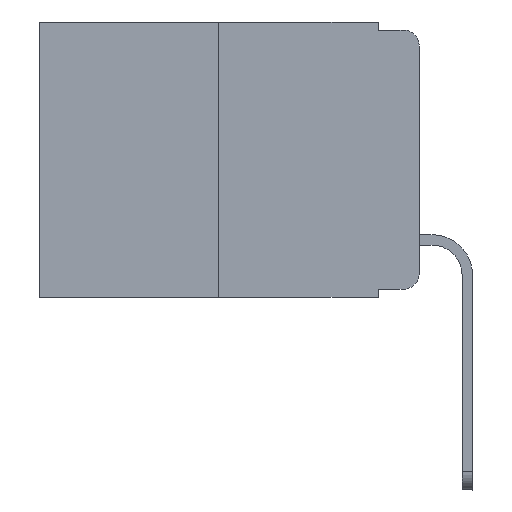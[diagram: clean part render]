
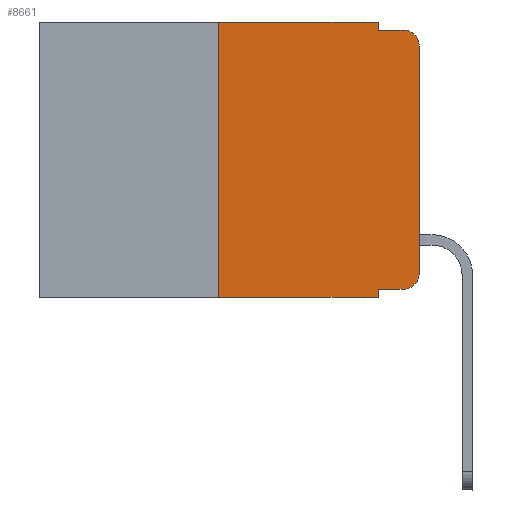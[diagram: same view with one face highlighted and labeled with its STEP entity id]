
A CAD part, left-side view. The second image highlights one B-rep face of the part: STEP entity #8661.
In plain terms, the highlighted planar face has unit normal (-1, 0, 0).
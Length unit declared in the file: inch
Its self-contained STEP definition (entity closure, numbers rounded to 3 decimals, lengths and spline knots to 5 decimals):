
#379 = EDGE_CURVE ( 'NONE', #13050, #4646, #15359, .T. ) ;
#973 = CARTESIAN_POINT ( 'NONE',  ( 0., 0., 0. ) ) ;
#1935 = ORIENTED_EDGE ( 'NONE', *, *, #5807, .F. ) ;
#2223 = ORIENTED_EDGE ( 'NONE', *, *, #12025, .T. ) ;
#2248 = CARTESIAN_POINT ( 'NONE',  ( 0., 0.051, -0.343 ) ) ;
#2332 = EDGE_CURVE ( 'NONE', #15812, #16675, #16079, .T. ) ;
#2363 = VERTEX_POINT ( 'NONE', #13544 ) ;
#3684 = EDGE_CURVE ( 'NONE', #21556, #7158, #5699, .T. ) ;
#3735 = CARTESIAN_POINT ( 'NONE',  ( 0., 0.473, 0. ) ) ;
#3888 = CARTESIAN_POINT ( 'NONE',  ( 0., 0.25, 0. ) ) ;
#4282 = VECTOR ( 'NONE', #18443, 39.37008 ) ;
#4646 = VERTEX_POINT ( 'NONE', #17001 ) ;
#5128 = CARTESIAN_POINT ( 'NONE',  ( 0., 0.25, -0.343 ) ) ;
#5597 = ORIENTED_EDGE ( 'NONE', *, *, #13949, .T. ) ;
#5699 = LINE ( 'NONE', #16818, #9567 ) ;
#5807 = EDGE_CURVE ( 'NONE', #2363, #13050, #10946, .T. ) ;
#5901 = CARTESIAN_POINT ( 'NONE',  ( 0., 0., -0.313 ) ) ;
#6930 = CIRCLE ( 'NONE', #9667, 0.02 ) ;
#7158 = VERTEX_POINT ( 'NONE', #9738 ) ;
#7371 = LINE ( 'NONE', #9457, #11361 ) ;
#7432 = DIRECTION ( 'NONE',  ( 0., 0., -1. ) ) ;
#7552 = DIRECTION ( 'NONE',  ( 0., 0., -1. ) ) ;
#8470 = VERTEX_POINT ( 'NONE', #10294 ) ;
#8509 = LINE ( 'NONE', #16039, #22608 ) ;
#8661 = ADVANCED_FACE ( 'NONE', ( #16834 ), #22338, .F. ) ;
#8668 = CARTESIAN_POINT ( 'NONE',  ( 0., 0.473, -0.343 ) ) ;
#9206 = ORIENTED_EDGE ( 'NONE', *, *, #379, .F. ) ;
#9457 = CARTESIAN_POINT ( 'NONE',  ( 0., 0.473, 0. ) ) ;
#9478 = VERTEX_POINT ( 'NONE', #3888 ) ;
#9567 = VECTOR ( 'NONE', #11366, 39.37008 ) ;
#9667 = AXIS2_PLACEMENT_3D ( 'NONE', #17781, #19611, #21569 ) ;
#9738 = CARTESIAN_POINT ( 'NONE',  ( 0., 0.02, -0.333 ) ) ;
#10294 = CARTESIAN_POINT ( 'NONE',  ( 0., 0., -0.03 ) ) ;
#10668 = VECTOR ( 'NONE', #16191, 39.37008 ) ;
#10749 = ORIENTED_EDGE ( 'NONE', *, *, #21478, .F. ) ;
#10913 = LINE ( 'NONE', #15093, #4282 ) ;
#10946 = LINE ( 'NONE', #16886, #16361 ) ;
#11163 = VECTOR ( 'NONE', #11833, 39.37008 ) ;
#11361 = VECTOR ( 'NONE', #14888, 39.37008 ) ;
#11366 = DIRECTION ( 'NONE',  ( 0., -1., 0. ) ) ;
#11609 = CARTESIAN_POINT ( 'NONE',  ( 0., 0.02, -0.313 ) ) ;
#11772 = DIRECTION ( 'NONE',  ( 0., -1., 0. ) ) ;
#11833 = DIRECTION ( 'NONE',  ( 0., 0., 1. ) ) ;
#12025 = EDGE_CURVE ( 'NONE', #7158, #15551, #13593, .T. ) ;
#12146 = CARTESIAN_POINT ( 'NONE',  ( 0., 0.051, -0.01 ) ) ;
#12442 = DIRECTION ( 'NONE',  ( 0., 0., 1. ) ) ;
#12834 = EDGE_CURVE ( 'NONE', #15812, #9478, #8509, .T. ) ;
#13050 = VERTEX_POINT ( 'NONE', #12146 ) ;
#13519 = VECTOR ( 'NONE', #11772, 39.37008 ) ;
#13544 = CARTESIAN_POINT ( 'NONE',  ( 0., 0.051, 0. ) ) ;
#13593 = CIRCLE ( 'NONE', #16760, 0.02 ) ;
#13949 = EDGE_CURVE ( 'NONE', #8470, #4646, #6930, .T. ) ;
#14345 = ORIENTED_EDGE ( 'NONE', *, *, #2332, .T. ) ;
#14888 = DIRECTION ( 'NONE',  ( 0., -1., 0. ) ) ;
#14961 = DIRECTION ( 'NONE',  ( 1., 0., 0. ) ) ;
#15014 = DIRECTION ( 'NONE',  ( 0., 0., -1. ) ) ;
#15093 = CARTESIAN_POINT ( 'NONE',  ( 0., 0.051, 0. ) ) ;
#15261 = EDGE_CURVE ( 'NONE', #15551, #8470, #15805, .T. ) ;
#15359 = LINE ( 'NONE', #22860, #13519 ) ;
#15551 = VERTEX_POINT ( 'NONE', #5901 ) ;
#15805 = LINE ( 'NONE', #973, #11163 ) ;
#15812 = VERTEX_POINT ( 'NONE', #5128 ) ;
#16039 = CARTESIAN_POINT ( 'NONE',  ( 0., 0.25, 0. ) ) ;
#16079 = LINE ( 'NONE', #8668, #10668 ) ;
#16191 = DIRECTION ( 'NONE',  ( 0., -1., 0. ) ) ;
#16223 = ORIENTED_EDGE ( 'NONE', *, *, #12834, .F. ) ;
#16361 = VECTOR ( 'NONE', #15014, 39.37008 ) ;
#16675 = VERTEX_POINT ( 'NONE', #2248 ) ;
#16760 = AXIS2_PLACEMENT_3D ( 'NONE', #11609, #17197, #7432 ) ;
#16818 = CARTESIAN_POINT ( 'NONE',  ( 0., 0.051, -0.333 ) ) ;
#16834 = FACE_OUTER_BOUND ( 'NONE', #23522, .T. ) ;
#16886 = CARTESIAN_POINT ( 'NONE',  ( 0., 0.051, 0. ) ) ;
#17001 = CARTESIAN_POINT ( 'NONE',  ( 0., 0.02, -0.01 ) ) ;
#17197 = DIRECTION ( 'NONE',  ( -1., 0., 0. ) ) ;
#17325 = ORIENTED_EDGE ( 'NONE', *, *, #3684, .T. ) ;
#17781 = CARTESIAN_POINT ( 'NONE',  ( 0., 0.02, -0.03 ) ) ;
#18443 = DIRECTION ( 'NONE',  ( 0., 0., -1. ) ) ;
#19611 = DIRECTION ( 'NONE',  ( -1., 0., 0. ) ) ;
#21279 = CARTESIAN_POINT ( 'NONE',  ( 0., 0.051, -0.333 ) ) ;
#21434 = ORIENTED_EDGE ( 'NONE', *, *, #21831, .F. ) ;
#21478 = EDGE_CURVE ( 'NONE', #9478, #2363, #7371, .T. ) ;
#21556 = VERTEX_POINT ( 'NONE', #21279 ) ;
#21569 = DIRECTION ( 'NONE',  ( 0., 0., -1. ) ) ;
#21831 = EDGE_CURVE ( 'NONE', #21556, #16675, #10913, .T. ) ;
#22338 = PLANE ( 'NONE',  #23315 ) ;
#22608 = VECTOR ( 'NONE', #12442, 39.37008 ) ;
#22732 = ORIENTED_EDGE ( 'NONE', *, *, #15261, .T. ) ;
#22860 = CARTESIAN_POINT ( 'NONE',  ( 0., 0.051, -0.01 ) ) ;
#23315 = AXIS2_PLACEMENT_3D ( 'NONE', #3735, #14961, #7552 ) ;
#23522 = EDGE_LOOP ( 'NONE', ( #22732, #5597, #9206, #1935, #10749, #16223, #14345, #21434, #17325, #2223 ) ) ;
